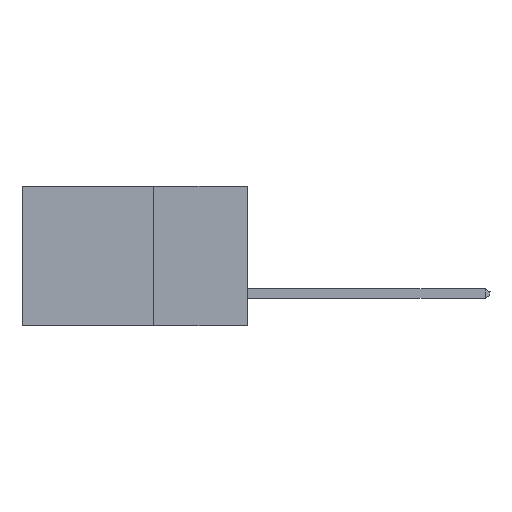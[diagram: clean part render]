
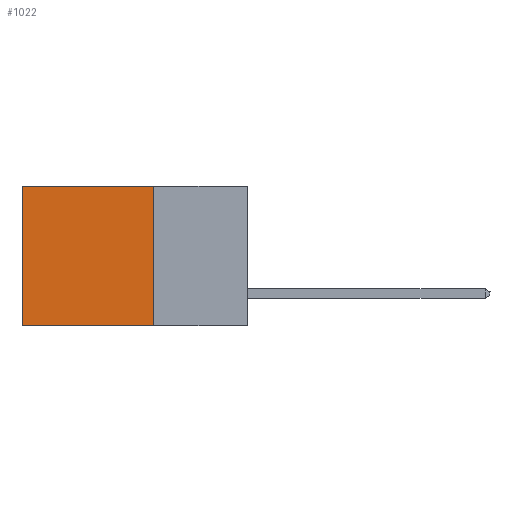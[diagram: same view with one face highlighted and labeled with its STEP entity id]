
A CAD part, left-side view. The second image highlights one B-rep face of the part: STEP entity #1022.
In plain terms, the highlighted planar face has unit normal (-1, 0, 0).
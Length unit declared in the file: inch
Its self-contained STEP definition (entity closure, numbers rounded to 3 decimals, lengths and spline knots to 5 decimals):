
#315 = VERTEX_POINT ( 'NONE', #9848 ) ;
#1022 = ADVANCED_FACE ( 'NONE', ( #4971 ), #17630, .F. ) ;
#1055 = EDGE_CURVE ( 'NONE', #315, #13125, #4558, .T. ) ;
#1188 = DIRECTION ( 'NONE',  ( 0., 0., -1. ) ) ;
#2261 = ORIENTED_EDGE ( 'NONE', *, *, #9240, .T. ) ;
#3187 = EDGE_CURVE ( 'NONE', #315, #20307, #18637, .T. ) ;
#4558 = LINE ( 'NONE', #14259, #20117 ) ;
#4765 = DIRECTION ( 'NONE',  ( 0., 1., 0. ) ) ;
#4971 = FACE_OUTER_BOUND ( 'NONE', #6713, .T. ) ;
#6713 = EDGE_LOOP ( 'NONE', ( #2261, #11179, #12103, #17985 ) ) ;
#8286 = LINE ( 'NONE', #11610, #17842 ) ;
#8707 = VERTEX_POINT ( 'NONE', #9547 ) ;
#8715 = LINE ( 'NONE', #13507, #16189 ) ;
#9240 = EDGE_CURVE ( 'NONE', #13125, #8707, #8286, .T. ) ;
#9547 = CARTESIAN_POINT ( 'NONE',  ( 0.2615, 0.6, -0.37 ) ) ;
#9848 = CARTESIAN_POINT ( 'NONE',  ( 0.2615, 0.25, 0. ) ) ;
#10413 = AXIS2_PLACEMENT_3D ( 'NONE', #14476, #20555, #16150 ) ;
#11179 = ORIENTED_EDGE ( 'NONE', *, *, #12011, .F. ) ;
#11320 = VECTOR ( 'NONE', #1188, 39.37008 ) ;
#11610 = CARTESIAN_POINT ( 'NONE',  ( 0.2615, 0.6, -0.37 ) ) ;
#12011 = EDGE_CURVE ( 'NONE', #20307, #8707, #8715, .T. ) ;
#12103 = ORIENTED_EDGE ( 'NONE', *, *, #3187, .F. ) ;
#12623 = CARTESIAN_POINT ( 'NONE',  ( 0.2615, 0.25, -0.37 ) ) ;
#12866 = DIRECTION ( 'NONE',  ( 0., 0., -1. ) ) ;
#13125 = VERTEX_POINT ( 'NONE', #16210 ) ;
#13507 = CARTESIAN_POINT ( 'NONE',  ( 0.2615, 0.25, -0.37 ) ) ;
#14259 = CARTESIAN_POINT ( 'NONE',  ( 0.2615, 0.25, 0. ) ) ;
#14476 = CARTESIAN_POINT ( 'NONE',  ( 0.2615, 0.25, -0.37 ) ) ;
#16150 = DIRECTION ( 'NONE',  ( 0., 0., -1. ) ) ;
#16189 = VECTOR ( 'NONE', #19922, 39.37008 ) ;
#16210 = CARTESIAN_POINT ( 'NONE',  ( 0.2615, 0.6, 0. ) ) ;
#17630 = PLANE ( 'NONE',  #10413 ) ;
#17842 = VECTOR ( 'NONE', #12866, 39.37008 ) ;
#17985 = ORIENTED_EDGE ( 'NONE', *, *, #1055, .T. ) ;
#18637 = LINE ( 'NONE', #20102, #11320 ) ;
#19922 = DIRECTION ( 'NONE',  ( 0., 1., 0. ) ) ;
#20102 = CARTESIAN_POINT ( 'NONE',  ( 0.2615, 0.25, -0.37 ) ) ;
#20117 = VECTOR ( 'NONE', #4765, 39.37008 ) ;
#20307 = VERTEX_POINT ( 'NONE', #12623 ) ;
#20555 = DIRECTION ( 'NONE',  ( 1., 0., 0. ) ) ;
